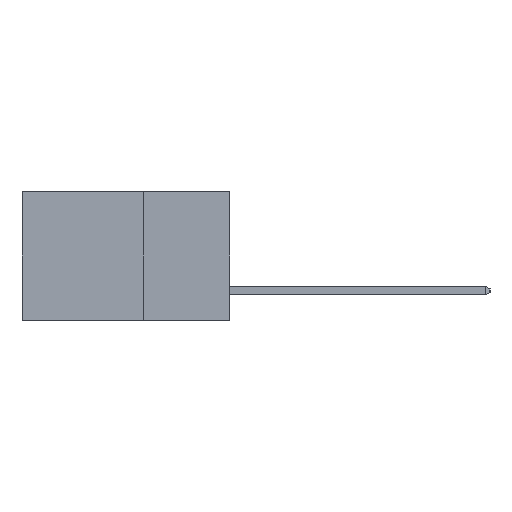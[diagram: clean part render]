
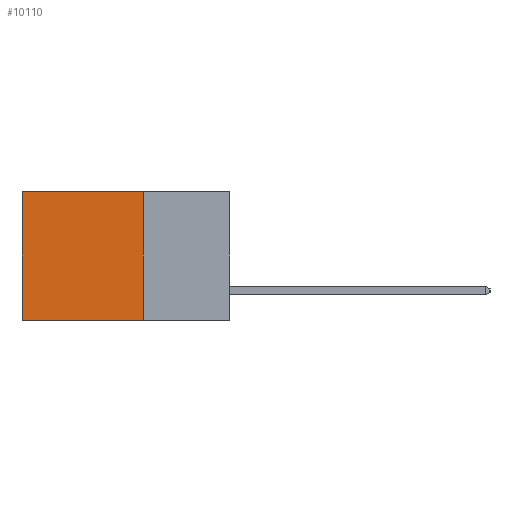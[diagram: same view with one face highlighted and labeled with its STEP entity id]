
A CAD part, left-side view. The second image highlights one B-rep face of the part: STEP entity #10110.
In plain terms, the highlighted planar face has unit normal (-1, 0, 0).
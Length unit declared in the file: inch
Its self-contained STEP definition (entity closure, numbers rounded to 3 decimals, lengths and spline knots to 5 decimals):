
#108 = LINE ( 'NONE', #21713, #4276 ) ;
#413 = ORIENTED_EDGE ( 'NONE', *, *, #10717, .T. ) ;
#1036 = EDGE_CURVE ( 'NONE', #16572, #25383, #4081, .T. ) ;
#1952 = CARTESIAN_POINT ( 'NONE',  ( 0.298, 0.25, 0. ) ) ;
#2416 = CARTESIAN_POINT ( 'NONE',  ( 0.298, 0.25, -0.37 ) ) ;
#3971 = FACE_OUTER_BOUND ( 'NONE', #12130, .T. ) ;
#4081 = LINE ( 'NONE', #10354, #14243 ) ;
#4188 = DIRECTION ( 'NONE',  ( 1., 0., 0. ) ) ;
#4276 = VECTOR ( 'NONE', #19768, 39.37008 ) ;
#4864 = EDGE_CURVE ( 'NONE', #19417, #13967, #18942, .T. ) ;
#5152 = CARTESIAN_POINT ( 'NONE',  ( 0.298, 0.6, -0.37 ) ) ;
#6696 = CARTESIAN_POINT ( 'NONE',  ( 0.298, 0.25, 0. ) ) ;
#6884 = CARTESIAN_POINT ( 'NONE',  ( 0.298, 0.6, 0. ) ) ;
#6961 = DIRECTION ( 'NONE',  ( 0., 0., -1. ) ) ;
#7963 = ORIENTED_EDGE ( 'NONE', *, *, #1036, .T. ) ;
#10110 = ADVANCED_FACE ( 'NONE', ( #3971 ), #16352, .F. ) ;
#10354 = CARTESIAN_POINT ( 'NONE',  ( 0.298, 0.6, 0. ) ) ;
#10717 = EDGE_CURVE ( 'NONE', #19417, #16572, #22333, .T. ) ;
#12058 = DIRECTION ( 'NONE',  ( 0., 1., 0. ) ) ;
#12130 = EDGE_LOOP ( 'NONE', ( #7963, #17100, #19072, #413 ) ) ;
#12172 = AXIS2_PLACEMENT_3D ( 'NONE', #12270, #4188, #18386 ) ;
#12270 = CARTESIAN_POINT ( 'NONE',  ( 0.298, 0.25, 0. ) ) ;
#12850 = CARTESIAN_POINT ( 'NONE',  ( 0.298, 0.25, 0. ) ) ;
#13967 = VERTEX_POINT ( 'NONE', #2416 ) ;
#14243 = VECTOR ( 'NONE', #6961, 39.37008 ) ;
#15685 = VECTOR ( 'NONE', #12058, 39.37008 ) ;
#16352 = PLANE ( 'NONE',  #12172 ) ;
#16572 = VERTEX_POINT ( 'NONE', #6884 ) ;
#16817 = EDGE_CURVE ( 'NONE', #13967, #25383, #108, .T. ) ;
#16900 = DIRECTION ( 'NONE',  ( 0., 0., -1. ) ) ;
#17100 = ORIENTED_EDGE ( 'NONE', *, *, #16817, .F. ) ;
#18386 = DIRECTION ( 'NONE',  ( 0., 0., -1. ) ) ;
#18942 = LINE ( 'NONE', #6696, #19575 ) ;
#19072 = ORIENTED_EDGE ( 'NONE', *, *, #4864, .F. ) ;
#19417 = VERTEX_POINT ( 'NONE', #12850 ) ;
#19575 = VECTOR ( 'NONE', #16900, 39.37008 ) ;
#19768 = DIRECTION ( 'NONE',  ( 0., 1., 0. ) ) ;
#21713 = CARTESIAN_POINT ( 'NONE',  ( 0.298, 0.25, -0.37 ) ) ;
#22333 = LINE ( 'NONE', #1952, #15685 ) ;
#25383 = VERTEX_POINT ( 'NONE', #5152 ) ;
